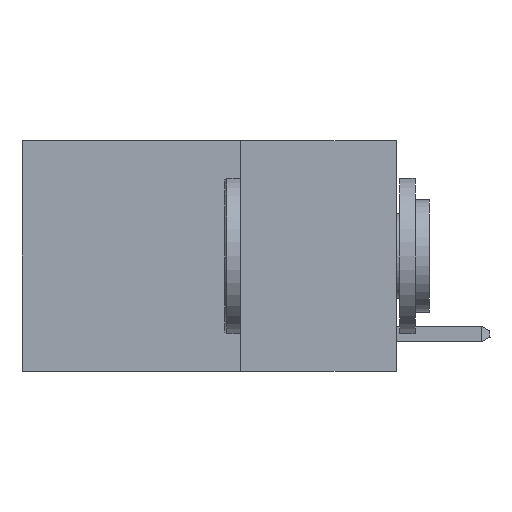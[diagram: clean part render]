
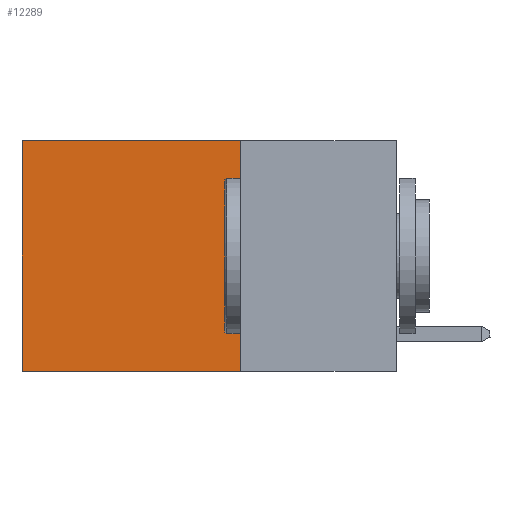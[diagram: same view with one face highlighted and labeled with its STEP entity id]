
A CAD part, left-side view. The second image highlights one B-rep face of the part: STEP entity #12289.
In plain terms, the highlighted planar face has unit normal (-1, 0, 0).
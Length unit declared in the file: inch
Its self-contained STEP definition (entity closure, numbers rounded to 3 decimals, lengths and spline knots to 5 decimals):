
#811 = EDGE_CURVE ( 'NONE', #1807, #18733, #19295, .T. ) ;
#881 = VERTEX_POINT ( 'NONE', #5769 ) ;
#1139 = DIRECTION ( 'NONE',  ( 0., 0., -1. ) ) ;
#1258 = CARTESIAN_POINT ( 'NONE',  ( 0.2625, 0.6, 0. ) ) ;
#1807 = VERTEX_POINT ( 'NONE', #18333 ) ;
#3009 = EDGE_CURVE ( 'NONE', #8603, #881, #4081, .T. ) ;
#3998 = CARTESIAN_POINT ( 'NONE',  ( 0.2625, 0.25, 0. ) ) ;
#4081 = LINE ( 'NONE', #10818, #12434 ) ;
#4720 = DIRECTION ( 'NONE',  ( 1., 0., 0. ) ) ;
#4985 = ORIENTED_EDGE ( 'NONE', *, *, #13611, .F. ) ;
#5336 = ORIENTED_EDGE ( 'NONE', *, *, #3009, .T. ) ;
#5769 = CARTESIAN_POINT ( 'NONE',  ( 0.2625, 0.6, 0. ) ) ;
#6564 = EDGE_CURVE ( 'NONE', #881, #18733, #9509, .T. ) ;
#8044 = VECTOR ( 'NONE', #14314, 39.37008 ) ;
#8177 = AXIS2_PLACEMENT_3D ( 'NONE', #14789, #4720, #16689 ) ;
#8603 = VERTEX_POINT ( 'NONE', #3998 ) ;
#9509 = LINE ( 'NONE', #1258, #16268 ) ;
#10818 = CARTESIAN_POINT ( 'NONE',  ( 0.2625, 0.25, 0. ) ) ;
#12289 = ADVANCED_FACE ( 'NONE', ( #14910 ), #18134, .F. ) ;
#12434 = VECTOR ( 'NONE', #17587, 39.37008 ) ;
#13611 = EDGE_CURVE ( 'NONE', #8603, #1807, #21008, .T. ) ;
#14241 = ORIENTED_EDGE ( 'NONE', *, *, #6564, .T. ) ;
#14314 = DIRECTION ( 'NONE',  ( 0., 1., 0. ) ) ;
#14789 = CARTESIAN_POINT ( 'NONE',  ( 0.2625, 0.25, 0. ) ) ;
#14880 = CARTESIAN_POINT ( 'NONE',  ( 0.2625, 0.6, -0.37 ) ) ;
#14910 = FACE_OUTER_BOUND ( 'NONE', #20166, .T. ) ;
#16151 = DIRECTION ( 'NONE',  ( 0., 0., -1. ) ) ;
#16268 = VECTOR ( 'NONE', #16151, 39.37008 ) ;
#16689 = DIRECTION ( 'NONE',  ( 0., 0., -1. ) ) ;
#17587 = DIRECTION ( 'NONE',  ( 0., 1., 0. ) ) ;
#17753 = CARTESIAN_POINT ( 'NONE',  ( 0.2625, 0.25, -0.37 ) ) ;
#18134 = PLANE ( 'NONE',  #8177 ) ;
#18333 = CARTESIAN_POINT ( 'NONE',  ( 0.2625, 0.25, -0.37 ) ) ;
#18733 = VERTEX_POINT ( 'NONE', #14880 ) ;
#19295 = LINE ( 'NONE', #17753, #8044 ) ;
#19870 = ORIENTED_EDGE ( 'NONE', *, *, #811, .F. ) ;
#19890 = VECTOR ( 'NONE', #1139, 39.37008 ) ;
#20166 = EDGE_LOOP ( 'NONE', ( #14241, #19870, #4985, #5336 ) ) ;
#20900 = CARTESIAN_POINT ( 'NONE',  ( 0.2625, 0.25, 0. ) ) ;
#21008 = LINE ( 'NONE', #20900, #19890 ) ;
